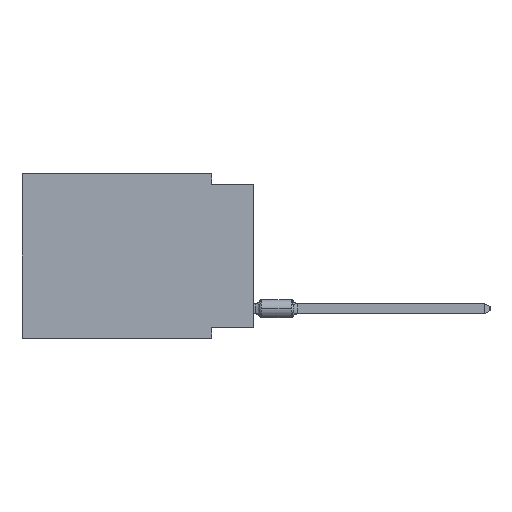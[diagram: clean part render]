
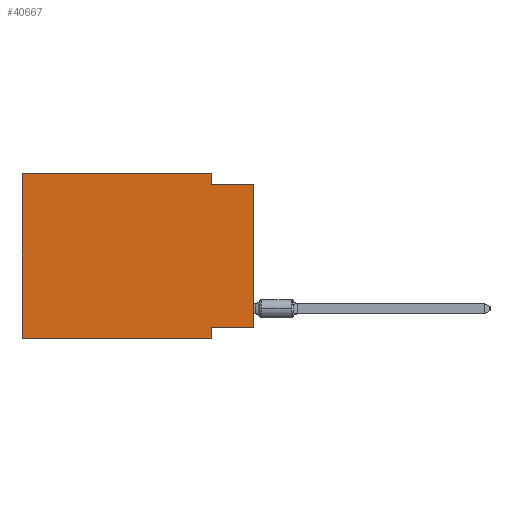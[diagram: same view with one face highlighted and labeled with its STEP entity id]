
A CAD part, left-side view. The second image highlights one B-rep face of the part: STEP entity #40667.
In plain terms, the highlighted planar face has unit normal (-1, 0, 0).
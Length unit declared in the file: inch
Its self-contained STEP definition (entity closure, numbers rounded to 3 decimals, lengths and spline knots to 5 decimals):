
#478 = DIRECTION ( 'NONE',  ( 0., 0., -1. ) ) ;
#1613 = ORIENTED_EDGE ( 'NONE', *, *, #24533, .F. ) ;
#1725 = LINE ( 'NONE', #20032, #28596 ) ;
#2164 = DIRECTION ( 'NONE',  ( 0., 1., 0. ) ) ;
#2239 = CARTESIAN_POINT ( 'NONE',  ( 0., 0.1, 0. ) ) ;
#2999 = EDGE_CURVE ( 'NONE', #22144, #21304, #37280, .T. ) ;
#3047 = LINE ( 'NONE', #42059, #10923 ) ;
#3355 = ORIENTED_EDGE ( 'NONE', *, *, #6080, .F. ) ;
#4217 = VERTEX_POINT ( 'NONE', #17644 ) ;
#6080 = EDGE_CURVE ( 'NONE', #38099, #4217, #16276, .T. ) ;
#6528 = VERTEX_POINT ( 'NONE', #8633 ) ;
#7923 = CARTESIAN_POINT ( 'NONE',  ( 0., 0., 0. ) ) ;
#8633 = CARTESIAN_POINT ( 'NONE',  ( 0., 0., -0.025 ) ) ;
#8693 = EDGE_CURVE ( 'NONE', #33461, #6528, #30032, .T. ) ;
#10651 = CARTESIAN_POINT ( 'NONE',  ( 0., 0.55, 0. ) ) ;
#10900 = CARTESIAN_POINT ( 'NONE',  ( 0., 0.1, -0.39 ) ) ;
#10923 = VECTOR ( 'NONE', #24927, 39.37008 ) ;
#11592 = ORIENTED_EDGE ( 'NONE', *, *, #15259, .T. ) ;
#12854 = LINE ( 'NONE', #20019, #27369 ) ;
#13566 = DIRECTION ( 'NONE',  ( 0., -1., 0. ) ) ;
#15259 = EDGE_CURVE ( 'NONE', #22144, #32833, #3047, .T. ) ;
#15643 = DIRECTION ( 'NONE',  ( 0., 0., 1. ) ) ;
#16276 = LINE ( 'NONE', #2239, #42946 ) ;
#16798 = VECTOR ( 'NONE', #27049, 39.37008 ) ;
#17644 = CARTESIAN_POINT ( 'NONE',  ( 0., 0.1, -0.025 ) ) ;
#17797 = LINE ( 'NONE', #10651, #33985 ) ;
#19696 = CARTESIAN_POINT ( 'NONE',  ( 0., 0.55, 0. ) ) ;
#20019 = CARTESIAN_POINT ( 'NONE',  ( 0., 0., -0.365 ) ) ;
#20032 = CARTESIAN_POINT ( 'NONE',  ( 0., 0., -0.025 ) ) ;
#20152 = LINE ( 'NONE', #34644, #16798 ) ;
#20311 = DIRECTION ( 'NONE',  ( 0., 0., -1. ) ) ;
#21304 = VERTEX_POINT ( 'NONE', #46381 ) ;
#21649 = CARTESIAN_POINT ( 'NONE',  ( 0., 0.55, 0. ) ) ;
#22144 = VERTEX_POINT ( 'NONE', #23102 ) ;
#22178 = ORIENTED_EDGE ( 'NONE', *, *, #44762, .F. ) ;
#23102 = CARTESIAN_POINT ( 'NONE',  ( 0., 0.55, -0.39 ) ) ;
#24533 = EDGE_CURVE ( 'NONE', #4217, #6528, #1725, .T. ) ;
#24927 = DIRECTION ( 'NONE',  ( 0., -1., 0. ) ) ;
#25162 = DIRECTION ( 'NONE',  ( 0., -1., 0. ) ) ;
#26541 = CARTESIAN_POINT ( 'NONE',  ( 0., 0., -0.365 ) ) ;
#26772 = EDGE_LOOP ( 'NONE', ( #29155, #1613, #3355, #37215, #43499, #11592, #39844, #22178 ) ) ;
#27049 = DIRECTION ( 'NONE',  ( 0., 0., -1. ) ) ;
#27369 = VECTOR ( 'NONE', #2164, 39.37008 ) ;
#27630 = PLANE ( 'NONE',  #27979 ) ;
#27979 = AXIS2_PLACEMENT_3D ( 'NONE', #21649, #32579, #478 ) ;
#28596 = VECTOR ( 'NONE', #13566, 39.37008 ) ;
#29155 = ORIENTED_EDGE ( 'NONE', *, *, #8693, .T. ) ;
#30032 = LINE ( 'NONE', #7923, #42669 ) ;
#31169 = FACE_OUTER_BOUND ( 'NONE', #26772, .T. ) ;
#31744 = EDGE_CURVE ( 'NONE', #37269, #32833, #20152, .T. ) ;
#32579 = DIRECTION ( 'NONE',  ( 1., 0., 0. ) ) ;
#32736 = CARTESIAN_POINT ( 'NONE',  ( 0., 0.1, -0.365 ) ) ;
#32833 = VERTEX_POINT ( 'NONE', #10900 ) ;
#33461 = VERTEX_POINT ( 'NONE', #26541 ) ;
#33983 = CARTESIAN_POINT ( 'NONE',  ( 0., 0.1, 0. ) ) ;
#33985 = VECTOR ( 'NONE', #25162, 39.37008 ) ;
#34644 = CARTESIAN_POINT ( 'NONE',  ( 0., 0.1, -0.39 ) ) ;
#37215 = ORIENTED_EDGE ( 'NONE', *, *, #39654, .F. ) ;
#37269 = VERTEX_POINT ( 'NONE', #32736 ) ;
#37280 = LINE ( 'NONE', #19696, #42391 ) ;
#38099 = VERTEX_POINT ( 'NONE', #33983 ) ;
#39654 = EDGE_CURVE ( 'NONE', #21304, #38099, #17797, .T. ) ;
#39844 = ORIENTED_EDGE ( 'NONE', *, *, #31744, .F. ) ;
#40667 = ADVANCED_FACE ( 'NONE', ( #31169 ), #27630, .F. ) ;
#42059 = CARTESIAN_POINT ( 'NONE',  ( 0., 0.55, -0.39 ) ) ;
#42391 = VECTOR ( 'NONE', #15643, 39.37008 ) ;
#42669 = VECTOR ( 'NONE', #43840, 39.37008 ) ;
#42946 = VECTOR ( 'NONE', #20311, 39.37008 ) ;
#43499 = ORIENTED_EDGE ( 'NONE', *, *, #2999, .F. ) ;
#43840 = DIRECTION ( 'NONE',  ( 0., 0., 1. ) ) ;
#44762 = EDGE_CURVE ( 'NONE', #33461, #37269, #12854, .T. ) ;
#46381 = CARTESIAN_POINT ( 'NONE',  ( 0., 0.55, 0. ) ) ;
